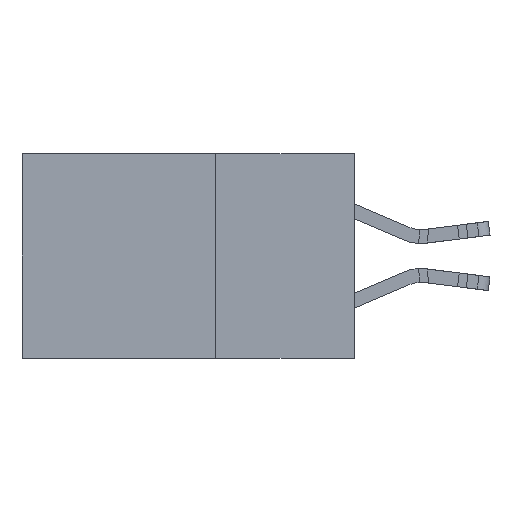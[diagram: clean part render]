
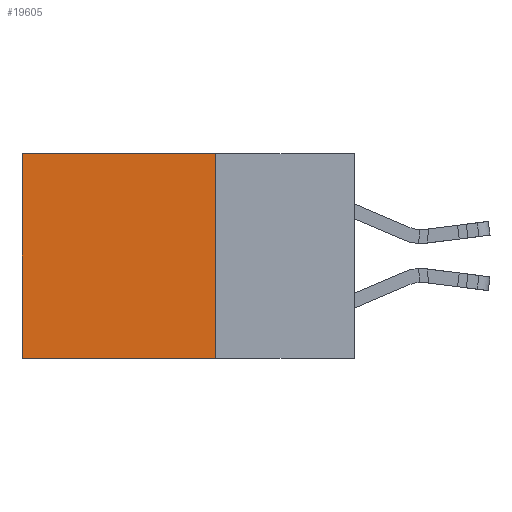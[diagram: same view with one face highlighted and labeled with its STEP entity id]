
A CAD part, left-side view. The second image highlights one B-rep face of the part: STEP entity #19605.
In plain terms, the highlighted planar face has unit normal (-1, 0, 0).
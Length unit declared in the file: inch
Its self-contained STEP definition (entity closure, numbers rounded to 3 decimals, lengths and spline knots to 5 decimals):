
#137 = CARTESIAN_POINT ( 'NONE',  ( 0.298, 0.25, 0. ) ) ;
#343 = LINE ( 'NONE', #20784, #1108 ) ;
#536 = EDGE_LOOP ( 'NONE', ( #19881, #21494, #14062, #21979 ) ) ;
#1108 = VECTOR ( 'NONE', #1290, 39.37008 ) ;
#1290 = DIRECTION ( 'NONE',  ( 0., 1., 0. ) ) ;
#1555 = LINE ( 'NONE', #137, #26083 ) ;
#4809 = DIRECTION ( 'NONE',  ( 0., 0., -1. ) ) ;
#5080 = DIRECTION ( 'NONE',  ( 0., 0., -1. ) ) ;
#5524 = VERTEX_POINT ( 'NONE', #25798 ) ;
#6623 = LINE ( 'NONE', #26831, #19643 ) ;
#11413 = CARTESIAN_POINT ( 'NONE',  ( 0.298, 0.25, 0. ) ) ;
#11771 = VERTEX_POINT ( 'NONE', #12018 ) ;
#12018 = CARTESIAN_POINT ( 'NONE',  ( 0.298, 0.25, 0. ) ) ;
#14062 = ORIENTED_EDGE ( 'NONE', *, *, #31227, .F. ) ;
#15089 = VECTOR ( 'NONE', #18763, 39.37008 ) ;
#15842 = LINE ( 'NONE', #11413, #15089 ) ;
#17007 = PLANE ( 'NONE',  #17256 ) ;
#17256 = AXIS2_PLACEMENT_3D ( 'NONE', #21829, #19471, #4809 ) ;
#17269 = EDGE_CURVE ( 'NONE', #5524, #18020, #343, .T. ) ;
#18020 = VERTEX_POINT ( 'NONE', #23538 ) ;
#18763 = DIRECTION ( 'NONE',  ( 0., 1., 0. ) ) ;
#19471 = DIRECTION ( 'NONE',  ( 1., 0., 0. ) ) ;
#19605 = ADVANCED_FACE ( 'NONE', ( #19845 ), #17007, .F. ) ;
#19643 = VECTOR ( 'NONE', #29258, 39.37008 ) ;
#19845 = FACE_OUTER_BOUND ( 'NONE', #536, .T. ) ;
#19881 = ORIENTED_EDGE ( 'NONE', *, *, #23364, .T. ) ;
#20514 = CARTESIAN_POINT ( 'NONE',  ( 0.298, 0.6, 0. ) ) ;
#20784 = CARTESIAN_POINT ( 'NONE',  ( 0.298, 0.25, -0.37 ) ) ;
#21494 = ORIENTED_EDGE ( 'NONE', *, *, #17269, .F. ) ;
#21829 = CARTESIAN_POINT ( 'NONE',  ( 0.298, 0.25, 0. ) ) ;
#21913 = EDGE_CURVE ( 'NONE', #11771, #28714, #15842, .T. ) ;
#21979 = ORIENTED_EDGE ( 'NONE', *, *, #21913, .T. ) ;
#23364 = EDGE_CURVE ( 'NONE', #28714, #18020, #6623, .T. ) ;
#23538 = CARTESIAN_POINT ( 'NONE',  ( 0.298, 0.6, -0.37 ) ) ;
#25798 = CARTESIAN_POINT ( 'NONE',  ( 0.298, 0.25, -0.37 ) ) ;
#26083 = VECTOR ( 'NONE', #5080, 39.37008 ) ;
#26831 = CARTESIAN_POINT ( 'NONE',  ( 0.298, 0.6, 0. ) ) ;
#28714 = VERTEX_POINT ( 'NONE', #20514 ) ;
#29258 = DIRECTION ( 'NONE',  ( 0., 0., -1. ) ) ;
#31227 = EDGE_CURVE ( 'NONE', #11771, #5524, #1555, .T. ) ;
